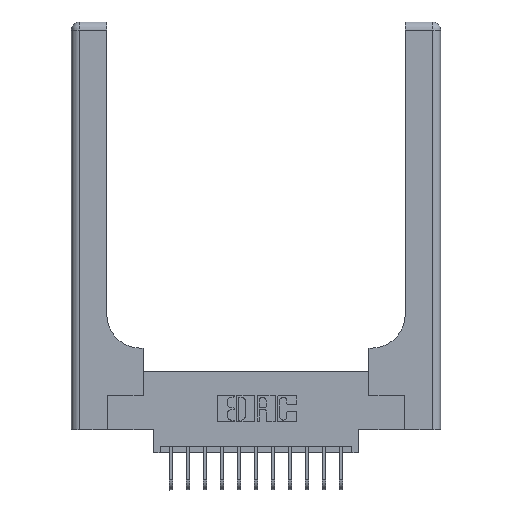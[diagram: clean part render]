
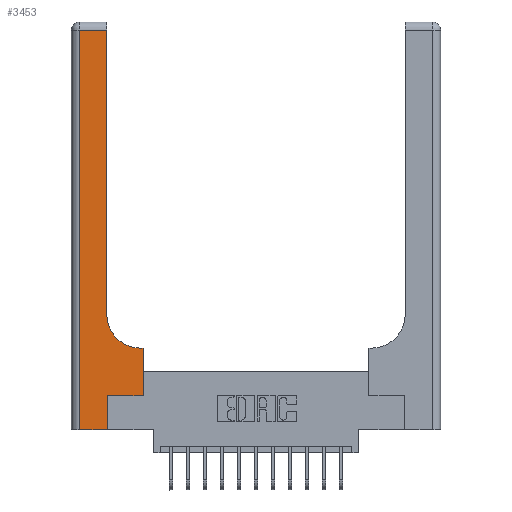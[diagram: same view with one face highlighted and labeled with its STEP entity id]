
A CAD part, top view. The second image highlights one B-rep face of the part: STEP entity #3453.
In plain terms, the highlighted planar face has unit normal (0, 0, 1).
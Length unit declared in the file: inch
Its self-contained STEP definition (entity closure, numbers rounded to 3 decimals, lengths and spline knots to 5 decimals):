
#190 = EDGE_CURVE ( 'NONE', #3768, #2922, #7224, .T. ) ;
#812 = ORIENTED_EDGE ( 'NONE', *, *, #7566, .T. ) ;
#850 = DIRECTION ( 'NONE',  ( 0., 1., 0. ) ) ;
#875 = DIRECTION ( 'NONE',  ( 0., 0., -1. ) ) ;
#905 = CARTESIAN_POINT ( 'NONE',  ( 0.528, 0.6, 0.37 ) ) ;
#949 = DIRECTION ( 'NONE',  ( 0., 1., 0. ) ) ;
#957 = CARTESIAN_POINT ( 'NONE',  ( 0.26, 0.6, 0.37 ) ) ;
#1018 = EDGE_CURVE ( 'NONE', #5896, #7101, #13103, .T. ) ;
#1696 = DIRECTION ( 'NONE',  ( -1., 0., 0. ) ) ;
#2009 = VECTOR ( 'NONE', #15948, 39.37008 ) ;
#2023 = EDGE_CURVE ( 'NONE', #3333, #3768, #10774, .T. ) ;
#2161 = CARTESIAN_POINT ( 'NONE',  ( 0.265, 0., 0.37 ) ) ;
#2277 = ORIENTED_EDGE ( 'NONE', *, *, #1018, .T. ) ;
#2382 = LINE ( 'NONE', #12504, #3022 ) ;
#2480 = FACE_OUTER_BOUND ( 'NONE', #4572, .T. ) ;
#2922 = VERTEX_POINT ( 'NONE', #905 ) ;
#2939 = ORIENTED_EDGE ( 'NONE', *, *, #6170, .T. ) ;
#3022 = VECTOR ( 'NONE', #850, 39.37008 ) ;
#3198 = CARTESIAN_POINT ( 'NONE',  ( 0.265, 0.25, 0.37 ) ) ;
#3333 = VERTEX_POINT ( 'NONE', #13790 ) ;
#3453 = ADVANCED_FACE ( 'NONE', ( #2480 ), #3741, .F. ) ;
#3741 = PLANE ( 'NONE',  #12662 ) ;
#3746 = CARTESIAN_POINT ( 'NONE',  ( 0.26, 2.94, 0.37 ) ) ;
#3768 = VERTEX_POINT ( 'NONE', #10102 ) ;
#3787 = VERTEX_POINT ( 'NONE', #7537 ) ;
#3949 = CARTESIAN_POINT ( 'NONE',  ( 0., 0., 0.37 ) ) ;
#4023 = DIRECTION ( 'NONE',  ( 1., 0., 0. ) ) ;
#4572 = EDGE_LOOP ( 'NONE', ( #2939, #2277, #14960, #812, #7604, #12586, #10944, #9129, #14138 ) ) ;
#4598 = VECTOR ( 'NONE', #949, 39.37008 ) ;
#4604 = VECTOR ( 'NONE', #8771, 39.37008 ) ;
#4679 = CARTESIAN_POINT ( 'NONE',  ( 0.528, 0.25, 0.37 ) ) ;
#5107 = DIRECTION ( 'NONE',  ( 0., 0., -1. ) ) ;
#5660 = VERTEX_POINT ( 'NONE', #2161 ) ;
#5896 = VERTEX_POINT ( 'NONE', #3746 ) ;
#6170 = EDGE_CURVE ( 'NONE', #3787, #5896, #16419, .T. ) ;
#6196 = EDGE_CURVE ( 'NONE', #2922, #11916, #8527, .T. ) ;
#6462 = CARTESIAN_POINT ( 'NONE',  ( 0., 2.94, 0.37 ) ) ;
#6977 = VECTOR ( 'NONE', #4023, 39.37008 ) ;
#7101 = VERTEX_POINT ( 'NONE', #7803 ) ;
#7224 = LINE ( 'NONE', #4679, #4598 ) ;
#7537 = CARTESIAN_POINT ( 'NONE',  ( 0.26, 0.85, 0.37 ) ) ;
#7566 = EDGE_CURVE ( 'NONE', #11111, #5660, #13046, .T. ) ;
#7604 = ORIENTED_EDGE ( 'NONE', *, *, #9729, .T. ) ;
#7709 = LINE ( 'NONE', #12895, #7890 ) ;
#7803 = CARTESIAN_POINT ( 'NONE',  ( 0.06, 2.94, 0.37 ) ) ;
#7864 = VECTOR ( 'NONE', #15204, 39.37008 ) ;
#7890 = VECTOR ( 'NONE', #10512, 39.37008 ) ;
#8492 = CIRCLE ( 'NONE', #14981, 0.25 ) ;
#8527 = LINE ( 'NONE', #957, #7864 ) ;
#8771 = DIRECTION ( 'NONE',  ( 0., 1., 0. ) ) ;
#9129 = ORIENTED_EDGE ( 'NONE', *, *, #6196, .T. ) ;
#9314 = EDGE_CURVE ( 'NONE', #11916, #3787, #8492, .T. ) ;
#9729 = EDGE_CURVE ( 'NONE', #5660, #3333, #2382, .T. ) ;
#9908 = CARTESIAN_POINT ( 'NONE',  ( 0.51, 0.6, 0.37 ) ) ;
#10102 = CARTESIAN_POINT ( 'NONE',  ( 0.528, 0.25, 0.37 ) ) ;
#10512 = DIRECTION ( 'NONE',  ( 0., -1., 0. ) ) ;
#10774 = LINE ( 'NONE', #3198, #2009 ) ;
#10944 = ORIENTED_EDGE ( 'NONE', *, *, #190, .T. ) ;
#11111 = VERTEX_POINT ( 'NONE', #13620 ) ;
#11455 = VECTOR ( 'NONE', #16840, 39.37008 ) ;
#11916 = VERTEX_POINT ( 'NONE', #9908 ) ;
#12504 = CARTESIAN_POINT ( 'NONE',  ( 0.265, 0., 0.37 ) ) ;
#12586 = ORIENTED_EDGE ( 'NONE', *, *, #2023, .T. ) ;
#12662 = AXIS2_PLACEMENT_3D ( 'NONE', #15382, #5107, #1696 ) ;
#12895 = CARTESIAN_POINT ( 'NONE',  ( 0.06, 3., 0.37 ) ) ;
#13046 = LINE ( 'NONE', #3949, #6977 ) ;
#13103 = LINE ( 'NONE', #6462, #11455 ) ;
#13342 = EDGE_CURVE ( 'NONE', #7101, #11111, #7709, .T. ) ;
#13620 = CARTESIAN_POINT ( 'NONE',  ( 0.06, 0., 0.37 ) ) ;
#13703 = CARTESIAN_POINT ( 'NONE',  ( 0.26, 3., 0.37 ) ) ;
#13790 = CARTESIAN_POINT ( 'NONE',  ( 0.265, 0.25, 0.37 ) ) ;
#14138 = ORIENTED_EDGE ( 'NONE', *, *, #9314, .T. ) ;
#14960 = ORIENTED_EDGE ( 'NONE', *, *, #13342, .T. ) ;
#14981 = AXIS2_PLACEMENT_3D ( 'NONE', #16676, #875, #15214 ) ;
#15204 = DIRECTION ( 'NONE',  ( -1., 0., 0. ) ) ;
#15214 = DIRECTION ( 'NONE',  ( 1., 0., 0. ) ) ;
#15382 = CARTESIAN_POINT ( 'NONE',  ( 0., 3., 0.37 ) ) ;
#15948 = DIRECTION ( 'NONE',  ( 1., 0., 0. ) ) ;
#16419 = LINE ( 'NONE', #13703, #4604 ) ;
#16676 = CARTESIAN_POINT ( 'NONE',  ( 0.51, 0.85, 0.37 ) ) ;
#16840 = DIRECTION ( 'NONE',  ( -1., 0., 0. ) ) ;
